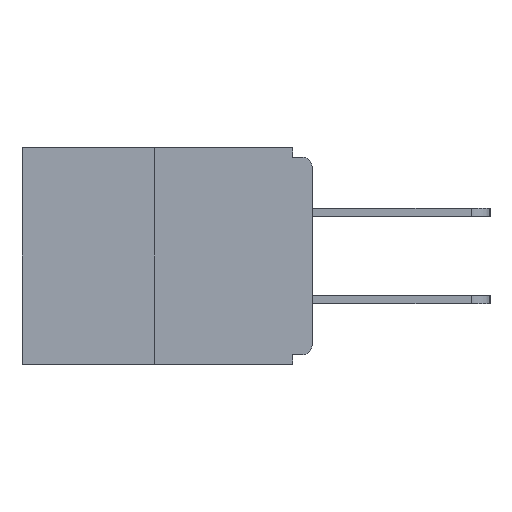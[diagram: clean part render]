
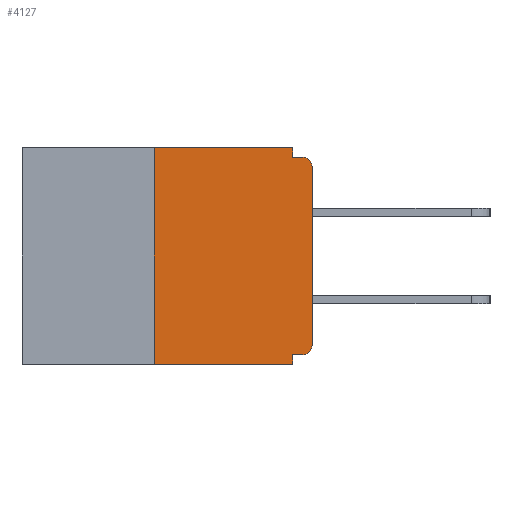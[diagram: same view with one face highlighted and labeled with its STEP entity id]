
A CAD part, left-side view. The second image highlights one B-rep face of the part: STEP entity #4127.
In plain terms, the highlighted planar face has unit normal (-1, 0, 0).
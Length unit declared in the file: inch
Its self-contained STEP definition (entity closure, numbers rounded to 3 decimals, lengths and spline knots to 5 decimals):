
#131 = DIRECTION ( 'NONE',  ( -1., 0., 0. ) ) ;
#179 = EDGE_CURVE ( 'NONE', #7869, #12963, #13206, .T. ) ;
#246 = CARTESIAN_POINT ( 'NONE',  ( 0., 0., -0.328 ) ) ;
#504 = ORIENTED_EDGE ( 'NONE', *, *, #16618, .F. ) ;
#1388 = VECTOR ( 'NONE', #13591, 39.37008 ) ;
#1503 = VERTEX_POINT ( 'NONE', #4540 ) ;
#1967 = DIRECTION ( 'NONE',  ( 0., 0., -1. ) ) ;
#2021 = ORIENTED_EDGE ( 'NONE', *, *, #16874, .F. ) ;
#2157 = CARTESIAN_POINT ( 'NONE',  ( 0., 0.46, 0. ) ) ;
#2276 = CARTESIAN_POINT ( 'NONE',  ( 0., 0.031, 0. ) ) ;
#2305 = DIRECTION ( 'NONE',  ( -1., 0., 0. ) ) ;
#2382 = EDGE_CURVE ( 'NONE', #12777, #1503, #16402, .T. ) ;
#2582 = CARTESIAN_POINT ( 'NONE',  ( 0., 0.031, 0. ) ) ;
#2752 = VECTOR ( 'NONE', #5592, 39.37008 ) ;
#2784 = CARTESIAN_POINT ( 'NONE',  ( 0., 0.25, 0. ) ) ;
#2806 = LINE ( 'NONE', #9770, #18984 ) ;
#2991 = VECTOR ( 'NONE', #18769, 39.37008 ) ;
#3040 = EDGE_CURVE ( 'NONE', #7869, #13794, #13471, .T. ) ;
#3414 = CARTESIAN_POINT ( 'NONE',  ( 0., 0., -0.015 ) ) ;
#3711 = DIRECTION ( 'NONE',  ( 0., 0., -1. ) ) ;
#4127 = ADVANCED_FACE ( 'NONE', ( #16628 ), #11403, .F. ) ;
#4178 = EDGE_CURVE ( 'NONE', #20796, #17620, #18223, .T. ) ;
#4540 = CARTESIAN_POINT ( 'NONE',  ( 0., 0., -0.03 ) ) ;
#5160 = ORIENTED_EDGE ( 'NONE', *, *, #4178, .F. ) ;
#5592 = DIRECTION ( 'NONE',  ( 0., -1., 0. ) ) ;
#6416 = CARTESIAN_POINT ( 'NONE',  ( 0., 0.46, 0. ) ) ;
#6936 = AXIS2_PLACEMENT_3D ( 'NONE', #2157, #10950, #9569 ) ;
#7232 = CARTESIAN_POINT ( 'NONE',  ( 0., 0., -0.313 ) ) ;
#7869 = VERTEX_POINT ( 'NONE', #8656 ) ;
#7926 = DIRECTION ( 'NONE',  ( 0., 0., -1. ) ) ;
#8656 = CARTESIAN_POINT ( 'NONE',  ( 0., 0.25, -0.343 ) ) ;
#8837 = CARTESIAN_POINT ( 'NONE',  ( 0., 0.031, -0.343 ) ) ;
#9569 = DIRECTION ( 'NONE',  ( 0., 0., -1. ) ) ;
#9770 = CARTESIAN_POINT ( 'NONE',  ( 0., 0.031, -0.343 ) ) ;
#10124 = VECTOR ( 'NONE', #11124, 39.37008 ) ;
#10341 = EDGE_CURVE ( 'NONE', #1503, #16614, #16512, .T. ) ;
#10545 = ORIENTED_EDGE ( 'NONE', *, *, #20292, .F. ) ;
#10857 = ORIENTED_EDGE ( 'NONE', *, *, #14202, .T. ) ;
#10950 = DIRECTION ( 'NONE',  ( 1., 0., 0. ) ) ;
#11124 = DIRECTION ( 'NONE',  ( 0., 1., 0. ) ) ;
#11244 = ORIENTED_EDGE ( 'NONE', *, *, #3040, .T. ) ;
#11337 = VECTOR ( 'NONE', #17260, 39.37008 ) ;
#11403 = PLANE ( 'NONE',  #6936 ) ;
#11485 = DIRECTION ( 'NONE',  ( 0., 0., -1. ) ) ;
#11503 = CARTESIAN_POINT ( 'NONE',  ( 0., 0.25, 0. ) ) ;
#11729 = CARTESIAN_POINT ( 'NONE',  ( 0., 0.46, -0.343 ) ) ;
#12055 = CARTESIAN_POINT ( 'NONE',  ( 0., 0.015, -0.313 ) ) ;
#12120 = VECTOR ( 'NONE', #7926, 39.37008 ) ;
#12626 = LINE ( 'NONE', #246, #10124 ) ;
#12777 = VERTEX_POINT ( 'NONE', #7232 ) ;
#12830 = AXIS2_PLACEMENT_3D ( 'NONE', #21374, #2305, #1967 ) ;
#12925 = DIRECTION ( 'NONE',  ( 0., 0., 1. ) ) ;
#12963 = VERTEX_POINT ( 'NONE', #11503 ) ;
#13206 = LINE ( 'NONE', #2784, #11337 ) ;
#13471 = LINE ( 'NONE', #11729, #2991 ) ;
#13591 = DIRECTION ( 'NONE',  ( 0., -1., 0. ) ) ;
#13794 = VERTEX_POINT ( 'NONE', #8837 ) ;
#14202 = EDGE_CURVE ( 'NONE', #19295, #12777, #22115, .T. ) ;
#15513 = ORIENTED_EDGE ( 'NONE', *, *, #10341, .T. ) ;
#15939 = EDGE_CURVE ( 'NONE', #19295, #20335, #12626, .T. ) ;
#16402 = LINE ( 'NONE', #19953, #19782 ) ;
#16512 = CIRCLE ( 'NONE', #12830, 0.015 ) ;
#16614 = VERTEX_POINT ( 'NONE', #17421 ) ;
#16618 = EDGE_CURVE ( 'NONE', #17620, #16614, #21433, .T. ) ;
#16621 = LINE ( 'NONE', #6416, #1388 ) ;
#16628 = FACE_OUTER_BOUND ( 'NONE', #19712, .T. ) ;
#16874 = EDGE_CURVE ( 'NONE', #20335, #13794, #2806, .T. ) ;
#17260 = DIRECTION ( 'NONE',  ( 0., 0., 1. ) ) ;
#17344 = AXIS2_PLACEMENT_3D ( 'NONE', #12055, #131, #3711 ) ;
#17421 = CARTESIAN_POINT ( 'NONE',  ( 0., 0.015, -0.015 ) ) ;
#17620 = VERTEX_POINT ( 'NONE', #19183 ) ;
#18223 = LINE ( 'NONE', #2276, #12120 ) ;
#18769 = DIRECTION ( 'NONE',  ( 0., -1., 0. ) ) ;
#18984 = VECTOR ( 'NONE', #11485, 39.37008 ) ;
#19183 = CARTESIAN_POINT ( 'NONE',  ( 0., 0.031, -0.015 ) ) ;
#19223 = CARTESIAN_POINT ( 'NONE',  ( 0., 0.015, -0.328 ) ) ;
#19285 = ORIENTED_EDGE ( 'NONE', *, *, #2382, .T. ) ;
#19295 = VERTEX_POINT ( 'NONE', #19223 ) ;
#19712 = EDGE_LOOP ( 'NONE', ( #10545, #20344, #11244, #2021, #22317, #10857, #19285, #15513, #504, #5160 ) ) ;
#19782 = VECTOR ( 'NONE', #12925, 39.37008 ) ;
#19953 = CARTESIAN_POINT ( 'NONE',  ( 0., 0., 0. ) ) ;
#20292 = EDGE_CURVE ( 'NONE', #12963, #20796, #16621, .T. ) ;
#20335 = VERTEX_POINT ( 'NONE', #22255 ) ;
#20344 = ORIENTED_EDGE ( 'NONE', *, *, #179, .F. ) ;
#20796 = VERTEX_POINT ( 'NONE', #2582 ) ;
#21374 = CARTESIAN_POINT ( 'NONE',  ( 0., 0.015, -0.03 ) ) ;
#21433 = LINE ( 'NONE', #3414, #2752 ) ;
#22115 = CIRCLE ( 'NONE', #17344, 0.015 ) ;
#22255 = CARTESIAN_POINT ( 'NONE',  ( 0., 0.031, -0.328 ) ) ;
#22317 = ORIENTED_EDGE ( 'NONE', *, *, #15939, .F. ) ;
